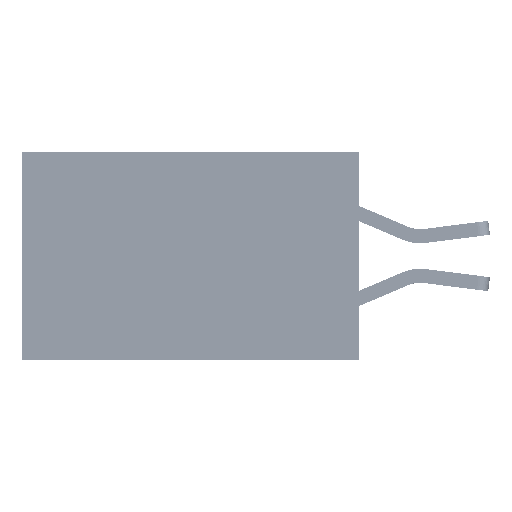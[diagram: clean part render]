
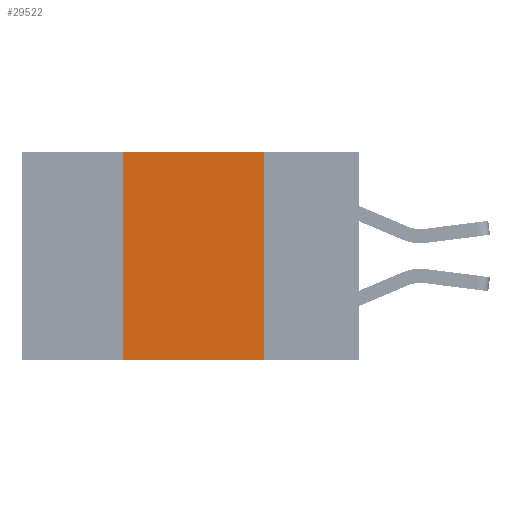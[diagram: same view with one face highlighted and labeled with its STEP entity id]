
A CAD part, left-side view. The second image highlights one B-rep face of the part: STEP entity #29522.
In plain terms, the highlighted planar face has unit normal (-1, 0, 0).
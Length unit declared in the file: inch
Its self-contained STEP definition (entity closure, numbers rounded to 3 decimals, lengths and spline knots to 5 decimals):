
#464 = ORIENTED_EDGE ( 'NONE', *, *, #33610, .F. ) ;
#2230 = CARTESIAN_POINT ( 'NONE',  ( 0., 0.6, 0. ) ) ;
#5035 = CARTESIAN_POINT ( 'NONE',  ( 0., 0.42, 0. ) ) ;
#5415 = DIRECTION ( 'NONE',  ( 0., 0., 1. ) ) ;
#6195 = VECTOR ( 'NONE', #13536, 39.37008 ) ;
#6833 = CARTESIAN_POINT ( 'NONE',  ( 0., 0.6, 0. ) ) ;
#7523 = DIRECTION ( 'NONE',  ( 0., 0., -1. ) ) ;
#11543 = ORIENTED_EDGE ( 'NONE', *, *, #21917, .T. ) ;
#11748 = CARTESIAN_POINT ( 'NONE',  ( 0., 0.42, 0. ) ) ;
#12254 = VERTEX_POINT ( 'NONE', #13164 ) ;
#12384 = VECTOR ( 'NONE', #18123, 39.37008 ) ;
#13135 = VERTEX_POINT ( 'NONE', #26607 ) ;
#13164 = CARTESIAN_POINT ( 'NONE',  ( 0., 0.17, 0. ) ) ;
#13536 = DIRECTION ( 'NONE',  ( 0., -1., 0. ) ) ;
#14074 = DIRECTION ( 'NONE',  ( 0., 0., -1. ) ) ;
#15351 = CARTESIAN_POINT ( 'NONE',  ( 0., 0.42, -0.37 ) ) ;
#15431 = EDGE_CURVE ( 'NONE', #12254, #13135, #25310, .T. ) ;
#15702 = VERTEX_POINT ( 'NONE', #15351 ) ;
#18123 = DIRECTION ( 'NONE',  ( 0., -1., 0. ) ) ;
#19366 = AXIS2_PLACEMENT_3D ( 'NONE', #2230, #30907, #14074 ) ;
#19472 = CARTESIAN_POINT ( 'NONE',  ( 0., 0.6, -0.37 ) ) ;
#19760 = LINE ( 'NONE', #5035, #28029 ) ;
#21745 = LINE ( 'NONE', #6833, #12384 ) ;
#21777 = LINE ( 'NONE', #19472, #6195 ) ;
#21917 = EDGE_CURVE ( 'NONE', #15702, #13135, #21777, .T. ) ;
#22624 = CARTESIAN_POINT ( 'NONE',  ( 0., 0.17, 0. ) ) ;
#22684 = FACE_OUTER_BOUND ( 'NONE', #31509, .T. ) ;
#23062 = PLANE ( 'NONE',  #19366 ) ;
#23753 = VERTEX_POINT ( 'NONE', #11748 ) ;
#25274 = EDGE_CURVE ( 'NONE', #23753, #12254, #21745, .T. ) ;
#25310 = LINE ( 'NONE', #22624, #27953 ) ;
#26607 = CARTESIAN_POINT ( 'NONE',  ( 0., 0.17, -0.37 ) ) ;
#27953 = VECTOR ( 'NONE', #7523, 39.37008 ) ;
#28029 = VECTOR ( 'NONE', #5415, 39.37008 ) ;
#29522 = ADVANCED_FACE ( 'NONE', ( #22684 ), #23062, .F. ) ;
#30907 = DIRECTION ( 'NONE',  ( 1., 0., 0. ) ) ;
#31509 = EDGE_LOOP ( 'NONE', ( #32022, #35837, #464, #11543 ) ) ;
#32022 = ORIENTED_EDGE ( 'NONE', *, *, #15431, .F. ) ;
#33610 = EDGE_CURVE ( 'NONE', #15702, #23753, #19760, .T. ) ;
#35837 = ORIENTED_EDGE ( 'NONE', *, *, #25274, .F. ) ;
